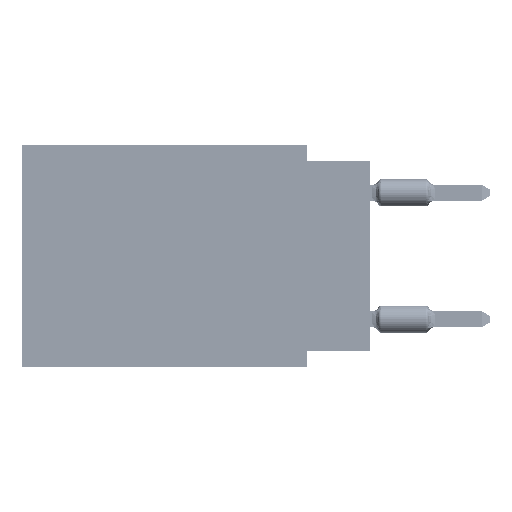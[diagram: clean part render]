
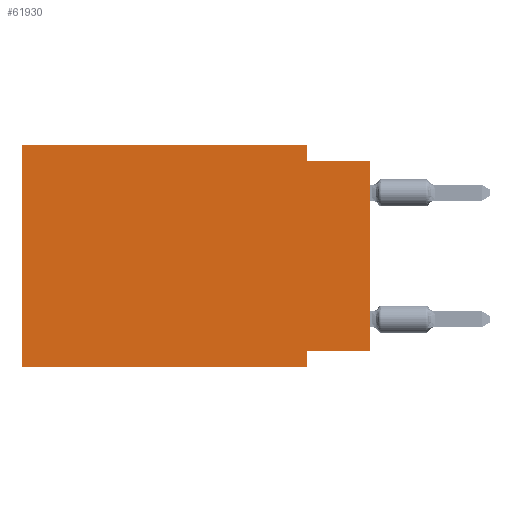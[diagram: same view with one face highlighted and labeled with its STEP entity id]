
A CAD part, left-side view. The second image highlights one B-rep face of the part: STEP entity #61930.
In plain terms, the highlighted planar face has unit normal (-1, 0, 0).
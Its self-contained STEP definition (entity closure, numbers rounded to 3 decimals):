
#248 = VERTEX_POINT ( 'NONE', #39860 ) ;
#252 = CARTESIAN_POINT ( 'NONE',  ( 0., 13.97, -8.89 ) ) ;
#5714 = VECTOR ( 'NONE', #64544, 1000. ) ;
#7792 = VECTOR ( 'NONE', #62267, 1000. ) ;
#8622 = VERTEX_POINT ( 'NONE', #252 ) ;
#10396 = CARTESIAN_POINT ( 'NONE',  ( 0., 13.97, -8.89 ) ) ;
#11133 = VERTEX_POINT ( 'NONE', #108514 ) ;
#11252 = EDGE_CURVE ( 'NONE', #84312, #248, #26294, .T. ) ;
#13032 = VERTEX_POINT ( 'NONE', #104875 ) ;
#17045 = ORIENTED_EDGE ( 'NONE', *, *, #67213, .F. ) ;
#17095 = LINE ( 'NONE', #33665, #35060 ) ;
#18353 = LINE ( 'NONE', #10396, #7792 ) ;
#21077 = CARTESIAN_POINT ( 'NONE',  ( 0., 0., -8.255 ) ) ;
#21929 = DIRECTION ( 'NONE',  ( 0., -1., 0. ) ) ;
#22473 = LINE ( 'NONE', #66381, #27641 ) ;
#26294 = LINE ( 'NONE', #61060, #28862 ) ;
#27105 = VECTOR ( 'NONE', #21929, 1000. ) ;
#27242 = CARTESIAN_POINT ( 'NONE',  ( 0., 13.97, 0. ) ) ;
#27641 = VECTOR ( 'NONE', #50362, 1000. ) ;
#28307 = ORIENTED_EDGE ( 'NONE', *, *, #104016, .F. ) ;
#28862 = VECTOR ( 'NONE', #95871, 1000. ) ;
#30887 = VECTOR ( 'NONE', #85905, 1000. ) ;
#33665 = CARTESIAN_POINT ( 'NONE',  ( 0., 0., 0. ) ) ;
#35060 = VECTOR ( 'NONE', #85587, 1000. ) ;
#39611 = EDGE_CURVE ( 'NONE', #13032, #42738, #65554, .T. ) ;
#39860 = CARTESIAN_POINT ( 'NONE',  ( 0., 0., -0.635 ) ) ;
#42738 = VERTEX_POINT ( 'NONE', #102839 ) ;
#44194 = PLANE ( 'NONE',  #45226 ) ;
#45136 = CARTESIAN_POINT ( 'NONE',  ( 0., 2.54, -0.635 ) ) ;
#45226 = AXIS2_PLACEMENT_3D ( 'NONE', #89245, #53298, #106359 ) ;
#46804 = ORIENTED_EDGE ( 'NONE', *, *, #107932, .F. ) ;
#49040 = ORIENTED_EDGE ( 'NONE', *, *, #52530, .F. ) ;
#50362 = DIRECTION ( 'NONE',  ( 0., 0., -1. ) ) ;
#51590 = EDGE_CURVE ( 'NONE', #8622, #58473, #18353, .T. ) ;
#52530 = EDGE_CURVE ( 'NONE', #42738, #58473, #22473, .T. ) ;
#53298 = DIRECTION ( 'NONE',  ( 1., 0., 0. ) ) ;
#54072 = ORIENTED_EDGE ( 'NONE', *, *, #51590, .T. ) ;
#57831 = LINE ( 'NONE', #109197, #27105 ) ;
#58473 = VERTEX_POINT ( 'NONE', #61756 ) ;
#61060 = CARTESIAN_POINT ( 'NONE',  ( 0., 0., -0.635 ) ) ;
#61756 = CARTESIAN_POINT ( 'NONE',  ( 0., 2.54, -8.89 ) ) ;
#61930 = ADVANCED_FACE ( 'NONE', ( #80136 ), #44194, .F. ) ;
#62267 = DIRECTION ( 'NONE',  ( 0., -1., 0. ) ) ;
#64544 = DIRECTION ( 'NONE',  ( 0., 0., -1. ) ) ;
#65554 = LINE ( 'NONE', #21077, #30887 ) ;
#66381 = CARTESIAN_POINT ( 'NONE',  ( 0., 2.54, -8.89 ) ) ;
#67213 = EDGE_CURVE ( 'NONE', #8622, #73057, #84617, .T. ) ;
#68725 = ORIENTED_EDGE ( 'NONE', *, *, #11252, .F. ) ;
#73057 = VERTEX_POINT ( 'NONE', #27242 ) ;
#77548 = EDGE_LOOP ( 'NONE', ( #108717, #68725, #46804, #28307, #17045, #54072, #49040, #101872 ) ) ;
#80136 = FACE_OUTER_BOUND ( 'NONE', #77548, .T. ) ;
#82795 = CARTESIAN_POINT ( 'NONE',  ( 0., 2.54, 0. ) ) ;
#83930 = LINE ( 'NONE', #82795, #5714 ) ;
#84312 = VERTEX_POINT ( 'NONE', #45136 ) ;
#84617 = LINE ( 'NONE', #85162, #91338 ) ;
#85162 = CARTESIAN_POINT ( 'NONE',  ( 0., 13.97, 0. ) ) ;
#85587 = DIRECTION ( 'NONE',  ( 0., 0., 1. ) ) ;
#85905 = DIRECTION ( 'NONE',  ( 0., 1., 0. ) ) ;
#89245 = CARTESIAN_POINT ( 'NONE',  ( 0., 13.97, 0. ) ) ;
#91338 = VECTOR ( 'NONE', #111420, 1000. ) ;
#95871 = DIRECTION ( 'NONE',  ( 0., -1., 0. ) ) ;
#100324 = EDGE_CURVE ( 'NONE', #13032, #248, #17095, .T. ) ;
#101872 = ORIENTED_EDGE ( 'NONE', *, *, #39611, .F. ) ;
#102839 = CARTESIAN_POINT ( 'NONE',  ( 0., 2.54, -8.255 ) ) ;
#104016 = EDGE_CURVE ( 'NONE', #73057, #11133, #57831, .T. ) ;
#104875 = CARTESIAN_POINT ( 'NONE',  ( 0., 0., -8.255 ) ) ;
#106359 = DIRECTION ( 'NONE',  ( 0., 0., -1. ) ) ;
#107932 = EDGE_CURVE ( 'NONE', #11133, #84312, #83930, .T. ) ;
#108514 = CARTESIAN_POINT ( 'NONE',  ( 0., 2.54, 0. ) ) ;
#108717 = ORIENTED_EDGE ( 'NONE', *, *, #100324, .T. ) ;
#109197 = CARTESIAN_POINT ( 'NONE',  ( 0., 13.97, 0. ) ) ;
#111420 = DIRECTION ( 'NONE',  ( 0., 0., 1. ) ) ;
